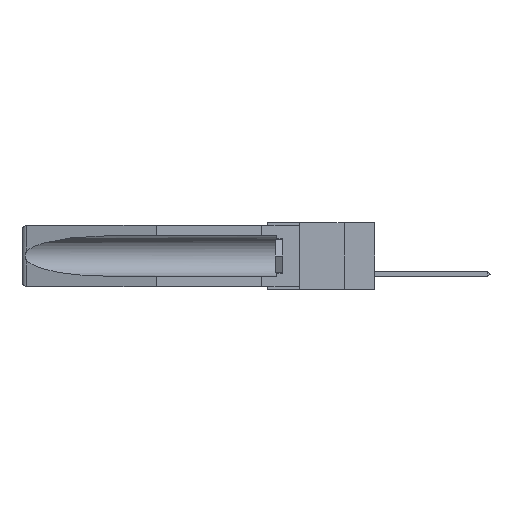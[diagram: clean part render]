
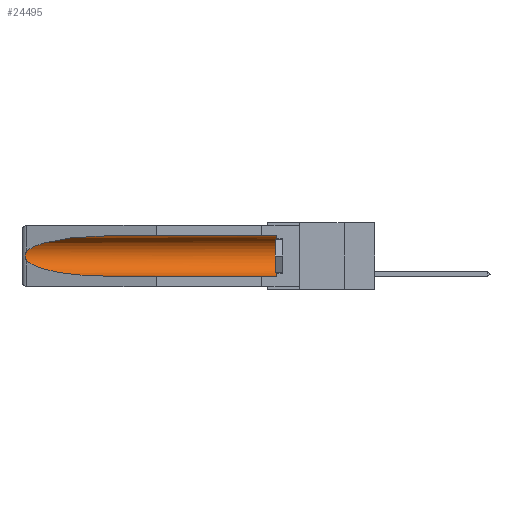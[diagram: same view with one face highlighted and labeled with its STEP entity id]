
A CAD part, left-side view. The second image highlights one B-rep face of the part: STEP entity #24495.
In plain terms, the highlighted cylindrical face has radius 2.857 mm (diameter 5.715 mm), a partial arc.
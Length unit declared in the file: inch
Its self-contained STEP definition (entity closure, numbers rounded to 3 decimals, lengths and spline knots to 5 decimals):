
#102 = AXIS2_PLACEMENT_3D ( 'NONE', #18991, #19083, #7789 ) ;
#422 = CARTESIAN_POINT ( 'NONE',  ( 0.155, 1.07973, -0.284 ) ) ;
#846 = CARTESIAN_POINT ( 'NONE',  ( 0.26537, 1.52718, -0.14972 ) ) ;
#847 = CARTESIAN_POINT ( 'NONE',  ( 0.25451, 1.48313, -0.24835 ) ) ;
#1449 = CARTESIAN_POINT ( 'NONE',  ( 0.155, 0.126, -0.284 ) ) ;
#1479 = ORIENTED_EDGE ( 'NONE', *, *, #9483, .T. ) ;
#2458 = CARTESIAN_POINT ( 'NONE',  ( 0.26537, 1.52718, -0.14972 ) ) ;
#2659 = CARTESIAN_POINT ( 'NONE',  ( 0.2673, 1.5327, -0.16383 ) ) ;
#4297 =( BOUNDED_CURVE ( )  B_SPLINE_CURVE ( 3, ( #21490, #16836, #14491, #846 ),
 .UNSPECIFIED., .F., .F. ) 
 B_SPLINE_CURVE_WITH_KNOTS ( ( 4, 4 ),
 ( 4.71239, 6.08839 ),
 .UNSPECIFIED. ) 
 CURVE ( )  GEOMETRIC_REPRESENTATION_ITEM ( )  RATIONAL_B_SPLINE_CURVE ( ( 1., 0.848, 0.848, 1. ) ) 
 REPRESENTATION_ITEM ( '' )  );
#4459 = EDGE_CURVE ( 'NONE', #7353, #6915, #21170, .T. ) ;
#4747 = CARTESIAN_POINT ( 'NONE',  ( 0.26597, 1.5296, -0.19026 ) ) ;
#4771 = VERTEX_POINT ( 'NONE', #15583 ) ;
#4938 = DIRECTION ( 'NONE',  ( 0., 0., 1. ) ) ;
#5417 = CARTESIAN_POINT ( 'NONE',  ( 0.26537, 1.52718, -0.19328 ) ) ;
#5884 = CARTESIAN_POINT ( 'NONE',  ( 0.155, -0.30754, -0.284 ) ) ;
#6815 = CARTESIAN_POINT ( 'NONE',  ( 0.26597, 1.52961, -0.15275 ) ) ;
#6915 = VERTEX_POINT ( 'NONE', #24536 ) ;
#6951 = CIRCLE ( 'NONE', #9001, 0.1125 ) ;
#7197 = ORIENTED_EDGE ( 'NONE', *, *, #13585, .T. ) ;
#7353 = VERTEX_POINT ( 'NONE', #17134 ) ;
#7789 = DIRECTION ( 'NONE',  ( 0., 0., 1. ) ) ;
#8419 = EDGE_CURVE ( 'NONE', #6915, #4771, #4297, .T. ) ;
#8571 = VERTEX_POINT ( 'NONE', #1449 ) ;
#8755 = LINE ( 'NONE', #5884, #29037 ) ;
#8959 = CARTESIAN_POINT ( 'NONE',  ( 0.26537, 1.52718, -0.19328 ) ) ;
#9001 = AXIS2_PLACEMENT_3D ( 'NONE', #16047, #16337, #4938 ) ;
#9163 = CARTESIAN_POINT ( 'NONE',  ( 0.26655, 1.53094, -0.18657 ) ) ;
#9245 = CYLINDRICAL_SURFACE ( 'NONE', #102, 0.1125 ) ;
#9262 = CARTESIAN_POINT ( 'NONE',  ( 0.2675, 1.53308, -0.17534 ) ) ;
#9483 = EDGE_CURVE ( 'NONE', #20698, #9904, #21003, .T. ) ;
#9904 = VERTEX_POINT ( 'NONE', #422 ) ;
#12081 = ORIENTED_EDGE ( 'NONE', *, *, #21013, .F. ) ;
#12423 = FACE_OUTER_BOUND ( 'NONE', #26029, .T. ) ;
#13195 = ORIENTED_EDGE ( 'NONE', *, *, #4459, .T. ) ;
#13460 = B_SPLINE_CURVE_WITH_KNOTS ( 'NONE', 3,
 ( #2458, #6815, #16133, #2659, #22907, #9262, #22701, #9163, #4747, #18348 ),
 .UNSPECIFIED., .F., .F.,
 ( 4, 2, 2, 2, 4 ),
 ( 0., 0.00029, 0.00058, 0.00087, 0.00117 ),
 .UNSPECIFIED. ) ;
#13585 = EDGE_CURVE ( 'NONE', #4771, #20698, #13460, .T. ) ;
#14491 = CARTESIAN_POINT ( 'NONE',  ( 0.25451, 1.48313, -0.09465 ) ) ;
#15153 = VECTOR ( 'NONE', #23624, 39.37008 ) ;
#15583 = CARTESIAN_POINT ( 'NONE',  ( 0.26537, 1.52718, -0.14972 ) ) ;
#16047 = CARTESIAN_POINT ( 'NONE',  ( 0.155, 0.126, -0.1715 ) ) ;
#16133 = CARTESIAN_POINT ( 'NONE',  ( 0.26654, 1.53092, -0.15636 ) ) ;
#16337 = DIRECTION ( 'NONE',  ( 0., -1., 0. ) ) ;
#16836 = CARTESIAN_POINT ( 'NONE',  ( 0.21114, 1.30732, -0.059 ) ) ;
#17134 = CARTESIAN_POINT ( 'NONE',  ( 0.155, 0.126, -0.059 ) ) ;
#17824 = EDGE_CURVE ( 'NONE', #8571, #7353, #6951, .T. ) ;
#18225 = ORIENTED_EDGE ( 'NONE', *, *, #17824, .T. ) ;
#18348 = CARTESIAN_POINT ( 'NONE',  ( 0.26537, 1.52718, -0.19328 ) ) ;
#18991 = CARTESIAN_POINT ( 'NONE',  ( 0.155, -0.30754, -0.1715 ) ) ;
#19015 = CARTESIAN_POINT ( 'NONE',  ( 0.21114, 1.30732, -0.284 ) ) ;
#19083 = DIRECTION ( 'NONE',  ( 0., 1., 0. ) ) ;
#20698 = VERTEX_POINT ( 'NONE', #8959 ) ;
#21003 =( BOUNDED_CURVE ( )  B_SPLINE_CURVE ( 3, ( #5417, #847, #19015, #25500 ),
 .UNSPECIFIED., .F., .F. ) 
 B_SPLINE_CURVE_WITH_KNOTS ( ( 4, 4 ),
 ( 0.1948, 1.5708 ),
 .UNSPECIFIED. ) 
 CURVE ( )  GEOMETRIC_REPRESENTATION_ITEM ( )  RATIONAL_B_SPLINE_CURVE ( ( 1., 0.848, 0.848, 1. ) ) 
 REPRESENTATION_ITEM ( '' )  );
#21013 = EDGE_CURVE ( 'NONE', #8571, #9904, #8755, .T. ) ;
#21170 = LINE ( 'NONE', #25945, #15153 ) ;
#21490 = CARTESIAN_POINT ( 'NONE',  ( 0.155, 1.07973, -0.059 ) ) ;
#22701 = CARTESIAN_POINT ( 'NONE',  ( 0.2673, 1.53269, -0.17917 ) ) ;
#22907 = CARTESIAN_POINT ( 'NONE',  ( 0.2675, 1.53308, -0.16763 ) ) ;
#23624 = DIRECTION ( 'NONE',  ( 0., 1., 0. ) ) ;
#24196 = DIRECTION ( 'NONE',  ( 0., 1., 0. ) ) ;
#24495 = ADVANCED_FACE ( 'NONE', ( #12423 ), #9245, .F. ) ;
#24536 = CARTESIAN_POINT ( 'NONE',  ( 0.155, 1.07973, -0.059 ) ) ;
#25317 = ORIENTED_EDGE ( 'NONE', *, *, #8419, .T. ) ;
#25500 = CARTESIAN_POINT ( 'NONE',  ( 0.155, 1.07973, -0.284 ) ) ;
#25945 = CARTESIAN_POINT ( 'NONE',  ( 0.155, -0.30754, -0.059 ) ) ;
#26029 = EDGE_LOOP ( 'NONE', ( #25317, #7197, #1479, #12081, #18225, #13195 ) ) ;
#29037 = VECTOR ( 'NONE', #24196, 39.37008 ) ;
